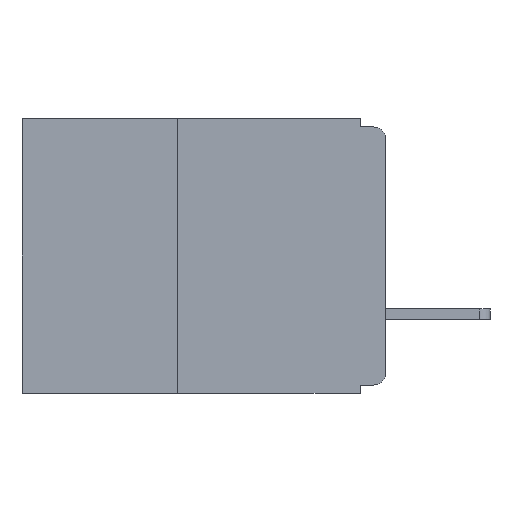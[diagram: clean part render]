
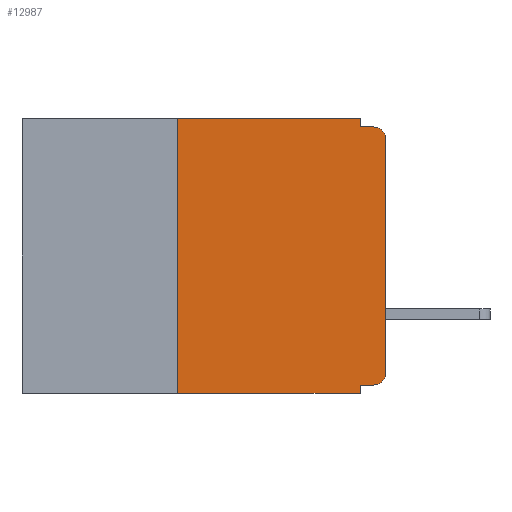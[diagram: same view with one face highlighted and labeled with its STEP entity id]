
A CAD part, left-side view. The second image highlights one B-rep face of the part: STEP entity #12987.
In plain terms, the highlighted planar face has unit normal (-1, 0, 0).
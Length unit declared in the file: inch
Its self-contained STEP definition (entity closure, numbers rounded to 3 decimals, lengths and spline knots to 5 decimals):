
#158 = VECTOR ( 'NONE', #3511, 39.37008 ) ;
#254 = CARTESIAN_POINT ( 'NONE',  ( 0., 0., 0. ) ) ;
#323 = VERTEX_POINT ( 'NONE', #9387 ) ;
#369 = DIRECTION ( 'NONE',  ( -1., 0., 0. ) ) ;
#740 = VERTEX_POINT ( 'NONE', #7019 ) ;
#807 = EDGE_LOOP ( 'NONE', ( #13295, #4986, #7537, #2006, #5525, #7402, #5950, #3580, #10714, #9442 ) ) ;
#1053 = DIRECTION ( 'NONE',  ( 0., -1., 0. ) ) ;
#1379 = DIRECTION ( 'NONE',  ( 0., 1., 0. ) ) ;
#2006 = ORIENTED_EDGE ( 'NONE', *, *, #9136, .F. ) ;
#2352 = CARTESIAN_POINT ( 'NONE',  ( 0., 0., -0.01 ) ) ;
#2588 = VERTEX_POINT ( 'NONE', #8031 ) ;
#2781 = VERTEX_POINT ( 'NONE', #13210 ) ;
#3203 = DIRECTION ( 'NONE',  ( 0., 0., 1. ) ) ;
#3244 = VERTEX_POINT ( 'NONE', #5080 ) ;
#3511 = DIRECTION ( 'NONE',  ( 0., -1., 0. ) ) ;
#3580 = ORIENTED_EDGE ( 'NONE', *, *, #9277, .F. ) ;
#3612 = AXIS2_PLACEMENT_3D ( 'NONE', #6045, #12744, #7100 ) ;
#3621 = VERTEX_POINT ( 'NONE', #5788 ) ;
#3645 = CIRCLE ( 'NONE', #3612, 0.015 ) ;
#3778 = VECTOR ( 'NONE', #11825, 39.37008 ) ;
#3869 = CARTESIAN_POINT ( 'NONE',  ( 0., 0.437, -0.33 ) ) ;
#4074 = VERTEX_POINT ( 'NONE', #13244 ) ;
#4364 = LINE ( 'NONE', #11004, #6520 ) ;
#4680 = CARTESIAN_POINT ( 'NONE',  ( 0., 0.437, 0. ) ) ;
#4797 = VERTEX_POINT ( 'NONE', #5411 ) ;
#4871 = CARTESIAN_POINT ( 'NONE',  ( 0., 0.031, 0. ) ) ;
#4986 = ORIENTED_EDGE ( 'NONE', *, *, #7378, .T. ) ;
#5080 = CARTESIAN_POINT ( 'NONE',  ( 0., 0.031, -0.32 ) ) ;
#5411 = CARTESIAN_POINT ( 'NONE',  ( 0., 0.25, 0. ) ) ;
#5525 = ORIENTED_EDGE ( 'NONE', *, *, #11612, .F. ) ;
#5788 = CARTESIAN_POINT ( 'NONE',  ( 0., 0.031, -0.01 ) ) ;
#5950 = ORIENTED_EDGE ( 'NONE', *, *, #9234, .T. ) ;
#5966 = VERTEX_POINT ( 'NONE', #10091 ) ;
#5968 = DIRECTION ( 'NONE',  ( 0., 0., 1. ) ) ;
#6045 = CARTESIAN_POINT ( 'NONE',  ( 0., 0.015, -0.025 ) ) ;
#6089 = DIRECTION ( 'NONE',  ( 0., 0., -1. ) ) ;
#6511 = DIRECTION ( 'NONE',  ( 0., 0., -1. ) ) ;
#6520 = VECTOR ( 'NONE', #1379, 39.37008 ) ;
#6598 = CARTESIAN_POINT ( 'NONE',  ( 0., 0.25, -0.33 ) ) ;
#7007 = EDGE_CURVE ( 'NONE', #2588, #5966, #11968, .T. ) ;
#7019 = CARTESIAN_POINT ( 'NONE',  ( 0., 0.015, -0.32 ) ) ;
#7070 = VERTEX_POINT ( 'NONE', #6598 ) ;
#7100 = DIRECTION ( 'NONE',  ( 0., 0., -1. ) ) ;
#7145 = EDGE_CURVE ( 'NONE', #3621, #4074, #9130, .T. ) ;
#7242 = CARTESIAN_POINT ( 'NONE',  ( 0., 0.015, -0.305 ) ) ;
#7343 = EDGE_CURVE ( 'NONE', #740, #3244, #4364, .T. ) ;
#7378 = EDGE_CURVE ( 'NONE', #5966, #4074, #3645, .T. ) ;
#7402 = ORIENTED_EDGE ( 'NONE', *, *, #9177, .F. ) ;
#7467 = EDGE_CURVE ( 'NONE', #740, #2588, #13113, .T. ) ;
#7537 = ORIENTED_EDGE ( 'NONE', *, *, #7145, .F. ) ;
#8031 = CARTESIAN_POINT ( 'NONE',  ( 0., 0., -0.305 ) ) ;
#8200 = CARTESIAN_POINT ( 'NONE',  ( 0., 0.031, -0.33 ) ) ;
#8337 = DIRECTION ( 'NONE',  ( 0., 0., -1. ) ) ;
#8599 = PLANE ( 'NONE',  #10351 ) ;
#9082 = LINE ( 'NONE', #4871, #3778 ) ;
#9130 = LINE ( 'NONE', #2352, #158 ) ;
#9135 = DIRECTION ( 'NONE',  ( 0., -1., 0. ) ) ;
#9136 = EDGE_CURVE ( 'NONE', #2781, #3621, #9082, .T. ) ;
#9177 = EDGE_CURVE ( 'NONE', #7070, #4797, #11573, .T. ) ;
#9234 = EDGE_CURVE ( 'NONE', #7070, #323, #13196, .T. ) ;
#9277 = EDGE_CURVE ( 'NONE', #3244, #323, #12965, .T. ) ;
#9387 = CARTESIAN_POINT ( 'NONE',  ( 0., 0.031, -0.33 ) ) ;
#9442 = ORIENTED_EDGE ( 'NONE', *, *, #7467, .T. ) ;
#9540 = VECTOR ( 'NONE', #3203, 39.37008 ) ;
#10091 = CARTESIAN_POINT ( 'NONE',  ( 0., 0., -0.025 ) ) ;
#10351 = AXIS2_PLACEMENT_3D ( 'NONE', #13038, #12295, #6511 ) ;
#10359 = LINE ( 'NONE', #4680, #12446 ) ;
#10403 = VECTOR ( 'NONE', #9135, 39.37008 ) ;
#10618 = FACE_OUTER_BOUND ( 'NONE', #807, .T. ) ;
#10714 = ORIENTED_EDGE ( 'NONE', *, *, #7343, .F. ) ;
#10962 = CARTESIAN_POINT ( 'NONE',  ( 0., 0.25, -0.33 ) ) ;
#11004 = CARTESIAN_POINT ( 'NONE',  ( 0., 0., -0.32 ) ) ;
#11016 = VECTOR ( 'NONE', #5968, 39.37008 ) ;
#11573 = LINE ( 'NONE', #10962, #11016 ) ;
#11612 = EDGE_CURVE ( 'NONE', #4797, #2781, #10359, .T. ) ;
#11825 = DIRECTION ( 'NONE',  ( 0., 0., -1. ) ) ;
#11968 = LINE ( 'NONE', #254, #9540 ) ;
#12295 = DIRECTION ( 'NONE',  ( 1., 0., 0. ) ) ;
#12415 = AXIS2_PLACEMENT_3D ( 'NONE', #7242, #369, #8337 ) ;
#12446 = VECTOR ( 'NONE', #1053, 39.37008 ) ;
#12495 = VECTOR ( 'NONE', #6089, 39.37008 ) ;
#12744 = DIRECTION ( 'NONE',  ( -1., 0., 0. ) ) ;
#12965 = LINE ( 'NONE', #8200, #12495 ) ;
#12987 = ADVANCED_FACE ( 'NONE', ( #10618 ), #8599, .F. ) ;
#13038 = CARTESIAN_POINT ( 'NONE',  ( 0., 0.437, 0. ) ) ;
#13113 = CIRCLE ( 'NONE', #12415, 0.015 ) ;
#13196 = LINE ( 'NONE', #3869, #10403 ) ;
#13210 = CARTESIAN_POINT ( 'NONE',  ( 0., 0.031, 0. ) ) ;
#13244 = CARTESIAN_POINT ( 'NONE',  ( 0., 0.015, -0.01 ) ) ;
#13295 = ORIENTED_EDGE ( 'NONE', *, *, #7007, .T. ) ;
